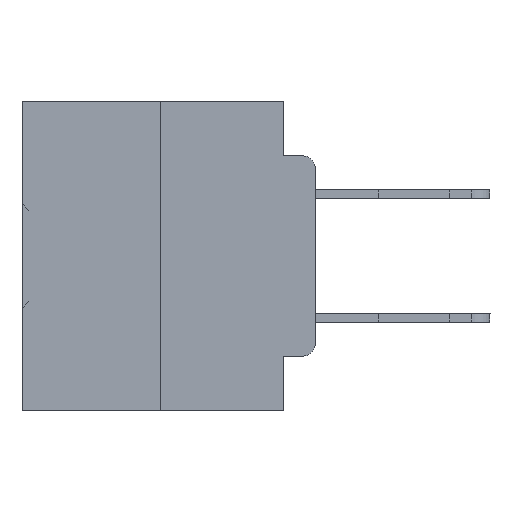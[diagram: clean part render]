
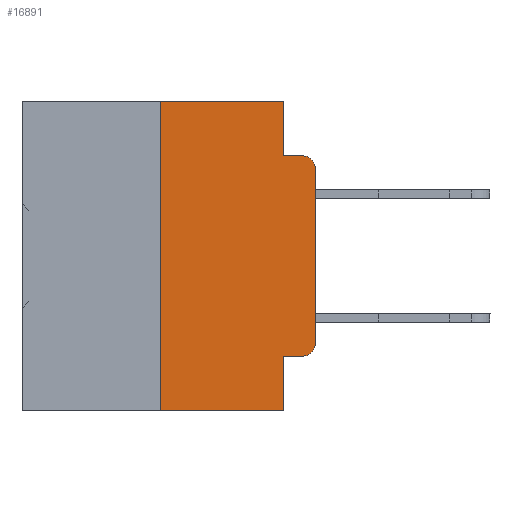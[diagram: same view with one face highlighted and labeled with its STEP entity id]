
A CAD part, left-side view. The second image highlights one B-rep face of the part: STEP entity #16891.
In plain terms, the highlighted planar face has unit normal (-1, 0, 0).
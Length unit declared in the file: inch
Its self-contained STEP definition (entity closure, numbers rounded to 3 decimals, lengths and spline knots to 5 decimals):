
#1185 = LINE ( 'NONE', #17560, #32068 ) ;
#1215 = LINE ( 'NONE', #27843, #23770 ) ;
#1332 = VERTEX_POINT ( 'NONE', #22292 ) ;
#1435 = CARTESIAN_POINT ( 'NONE',  ( 0., 0.051, 0. ) ) ;
#2013 = VECTOR ( 'NONE', #4215, 39.37008 ) ;
#2087 = DIRECTION ( 'NONE',  ( 0., -1., 0. ) ) ;
#2680 = VECTOR ( 'NONE', #14219, 39.37008 ) ;
#3013 = DIRECTION ( 'NONE',  ( -1., 0., 0. ) ) ;
#3272 = ORIENTED_EDGE ( 'NONE', *, *, #20579, .F. ) ;
#3341 = EDGE_CURVE ( 'NONE', #19719, #19577, #29160, .T. ) ;
#3917 = DIRECTION ( 'NONE',  ( 0., 0., 1. ) ) ;
#4033 = DIRECTION ( 'NONE',  ( 0., 0., -1. ) ) ;
#4034 = LINE ( 'NONE', #29704, #2680 ) ;
#4142 = ORIENTED_EDGE ( 'NONE', *, *, #13797, .T. ) ;
#4215 = DIRECTION ( 'NONE',  ( 0., -1., 0. ) ) ;
#4501 = VECTOR ( 'NONE', #4033, 39.37008 ) ;
#4504 = CARTESIAN_POINT ( 'NONE',  ( 0., 0.051, -0.4115 ) ) ;
#4695 = VERTEX_POINT ( 'NONE', #30197 ) ;
#5654 = ORIENTED_EDGE ( 'NONE', *, *, #36021, .F. ) ;
#5988 = DIRECTION ( 'NONE',  ( 0., 0., -1. ) ) ;
#6201 = EDGE_CURVE ( 'NONE', #19719, #20299, #1215, .T. ) ;
#7716 = CIRCLE ( 'NONE', #14545, 0.02 ) ;
#8508 = DIRECTION ( 'NONE',  ( -1., 0., 0. ) ) ;
#8906 = VERTEX_POINT ( 'NONE', #17672 ) ;
#10028 = ORIENTED_EDGE ( 'NONE', *, *, #31910, .T. ) ;
#11824 = LINE ( 'NONE', #1435, #4501 ) ;
#12206 = EDGE_CURVE ( 'NONE', #16474, #24699, #29053, .T. ) ;
#12898 = CARTESIAN_POINT ( 'NONE',  ( 0., 0., -0.1085 ) ) ;
#13048 = CARTESIAN_POINT ( 'NONE',  ( 0., 0.473, -0.5 ) ) ;
#13797 = EDGE_CURVE ( 'NONE', #37848, #1332, #7716, .T. ) ;
#14070 = DIRECTION ( 'NONE',  ( 0., -1., 0. ) ) ;
#14219 = DIRECTION ( 'NONE',  ( 0., 0., -1. ) ) ;
#14390 = ORIENTED_EDGE ( 'NONE', *, *, #6201, .F. ) ;
#14545 = AXIS2_PLACEMENT_3D ( 'NONE', #32087, #8508, #29147 ) ;
#14895 = CARTESIAN_POINT ( 'NONE',  ( 0., 0., -0.3915 ) ) ;
#15067 = CARTESIAN_POINT ( 'NONE',  ( 0., 0.02, -0.3915 ) ) ;
#15290 = CARTESIAN_POINT ( 'NONE',  ( 0., 0.051, -0.5 ) ) ;
#16474 = VERTEX_POINT ( 'NONE', #19582 ) ;
#16772 = DIRECTION ( 'NONE',  ( 0., 0., -1. ) ) ;
#16891 = ADVANCED_FACE ( 'NONE', ( #27324 ), #22563, .F. ) ;
#17560 = CARTESIAN_POINT ( 'NONE',  ( 0., 0.051, -0.0885 ) ) ;
#17672 = CARTESIAN_POINT ( 'NONE',  ( 0., 0.051, 0. ) ) ;
#18318 = AXIS2_PLACEMENT_3D ( 'NONE', #25500, #34650, #16772 ) ;
#19160 = ORIENTED_EDGE ( 'NONE', *, *, #29215, .F. ) ;
#19243 = DIRECTION ( 'NONE',  ( 0., -1., 0. ) ) ;
#19577 = VERTEX_POINT ( 'NONE', #15290 ) ;
#19582 = CARTESIAN_POINT ( 'NONE',  ( 0., 0.02, -0.4115 ) ) ;
#19719 = VERTEX_POINT ( 'NONE', #25913 ) ;
#20299 = VERTEX_POINT ( 'NONE', #31117 ) ;
#20368 = ORIENTED_EDGE ( 'NONE', *, *, #32458, .T. ) ;
#20579 = EDGE_CURVE ( 'NONE', #4695, #1332, #1185, .T. ) ;
#21238 = VECTOR ( 'NONE', #14070, 39.37008 ) ;
#21521 = CARTESIAN_POINT ( 'NONE',  ( 0., 0., 0. ) ) ;
#22173 = DIRECTION ( 'NONE',  ( 0., 0., 1. ) ) ;
#22292 = CARTESIAN_POINT ( 'NONE',  ( 0., 0.02, -0.0885 ) ) ;
#22563 = PLANE ( 'NONE',  #18318 ) ;
#23770 = VECTOR ( 'NONE', #22173, 39.37008 ) ;
#24699 = VERTEX_POINT ( 'NONE', #14895 ) ;
#25500 = CARTESIAN_POINT ( 'NONE',  ( 0., 0.473, 0. ) ) ;
#25913 = CARTESIAN_POINT ( 'NONE',  ( 0., 0.25, -0.5 ) ) ;
#26039 = EDGE_CURVE ( 'NONE', #8906, #4695, #11824, .T. ) ;
#26044 = CARTESIAN_POINT ( 'NONE',  ( 0., 0.473, 0. ) ) ;
#27324 = FACE_OUTER_BOUND ( 'NONE', #29699, .T. ) ;
#27766 = LINE ( 'NONE', #21521, #33720 ) ;
#27843 = CARTESIAN_POINT ( 'NONE',  ( 0., 0.25, 0. ) ) ;
#29053 = CIRCLE ( 'NONE', #29100, 0.02 ) ;
#29100 = AXIS2_PLACEMENT_3D ( 'NONE', #15067, #3013, #5988 ) ;
#29147 = DIRECTION ( 'NONE',  ( 0., 0., -1. ) ) ;
#29160 = LINE ( 'NONE', #13048, #2013 ) ;
#29215 = EDGE_CURVE ( 'NONE', #20299, #8906, #35074, .T. ) ;
#29699 = EDGE_LOOP ( 'NONE', ( #20368, #4142, #3272, #32523, #19160, #14390, #31604, #5654, #10028, #37670 ) ) ;
#29704 = CARTESIAN_POINT ( 'NONE',  ( 0., 0.051, 0. ) ) ;
#30083 = LINE ( 'NONE', #4504, #34687 ) ;
#30197 = CARTESIAN_POINT ( 'NONE',  ( 0., 0.051, -0.0885 ) ) ;
#30264 = VERTEX_POINT ( 'NONE', #31736 ) ;
#31117 = CARTESIAN_POINT ( 'NONE',  ( 0., 0.25, 0. ) ) ;
#31604 = ORIENTED_EDGE ( 'NONE', *, *, #3341, .T. ) ;
#31736 = CARTESIAN_POINT ( 'NONE',  ( 0., 0.051, -0.4115 ) ) ;
#31910 = EDGE_CURVE ( 'NONE', #30264, #16474, #30083, .T. ) ;
#32068 = VECTOR ( 'NONE', #2087, 39.37008 ) ;
#32087 = CARTESIAN_POINT ( 'NONE',  ( 0., 0.02, -0.1085 ) ) ;
#32458 = EDGE_CURVE ( 'NONE', #24699, #37848, #27766, .T. ) ;
#32523 = ORIENTED_EDGE ( 'NONE', *, *, #26039, .F. ) ;
#33720 = VECTOR ( 'NONE', #3917, 39.37008 ) ;
#34650 = DIRECTION ( 'NONE',  ( 1., 0., 0. ) ) ;
#34687 = VECTOR ( 'NONE', #19243, 39.37008 ) ;
#35074 = LINE ( 'NONE', #26044, #21238 ) ;
#36021 = EDGE_CURVE ( 'NONE', #30264, #19577, #4034, .T. ) ;
#37670 = ORIENTED_EDGE ( 'NONE', *, *, #12206, .T. ) ;
#37848 = VERTEX_POINT ( 'NONE', #12898 ) ;
